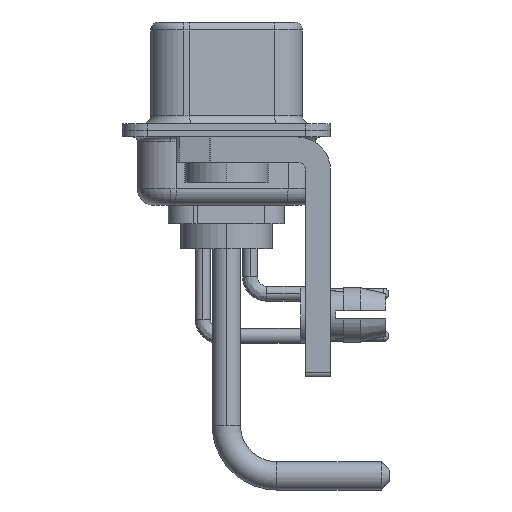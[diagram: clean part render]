
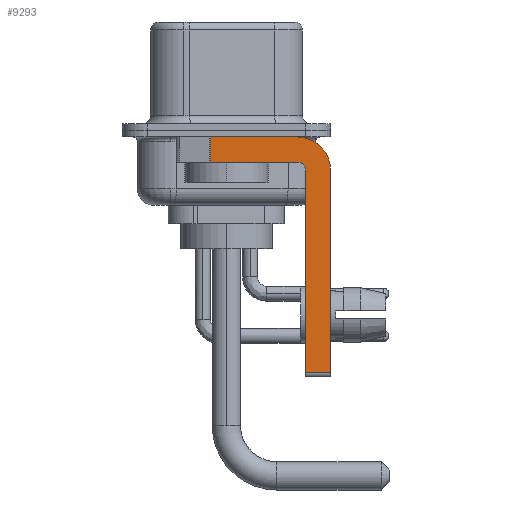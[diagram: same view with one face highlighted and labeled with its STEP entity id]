
A CAD part, left-side view. The second image highlights one B-rep face of the part: STEP entity #9293.
In plain terms, the highlighted planar face has unit normal (-1, 0, 0).
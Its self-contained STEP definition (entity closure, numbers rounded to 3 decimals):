
#61 = EDGE_CURVE ( 'NONE', #10969, #11477, #388, .T. ) ;
#388 = CIRCLE ( 'NONE', #13683, 2. ) ;
#877 = EDGE_CURVE ( 'NONE', #21684, #4207, #8972, .T. ) ;
#1241 = VERTEX_POINT ( 'NONE', #18661 ) ;
#1618 = CARTESIAN_POINT ( 'NONE',  ( -2.9, 0.978, -1.9 ) ) ;
#1762 = CARTESIAN_POINT ( 'NONE',  ( -2.9, -4.75, -14.8 ) ) ;
#1951 = DIRECTION ( 'NONE',  ( 1., 0., 0. ) ) ;
#2374 = VECTOR ( 'NONE', #17192, 1000. ) ;
#2614 = CIRCLE ( 'NONE', #9838, 0.5 ) ;
#2779 = DIRECTION ( 'NONE',  ( 1., 0., 0. ) ) ;
#2780 = DIRECTION ( 'NONE',  ( 0., 1., 0. ) ) ;
#2795 = EDGE_LOOP ( 'NONE', ( #20848, #18134, #19923, #14356, #10667, #23941, #11765, #3716 ) ) ;
#2895 = EDGE_CURVE ( 'NONE', #1241, #10969, #12571, .T. ) ;
#2924 = VERTEX_POINT ( 'NONE', #18760 ) ;
#3509 = LINE ( 'NONE', #1618, #22342 ) ;
#3649 = VECTOR ( 'NONE', #8600, 1000. ) ;
#3716 = ORIENTED_EDGE ( 'NONE', *, *, #61, .F. ) ;
#4207 = VERTEX_POINT ( 'NONE', #20794 ) ;
#4671 = PLANE ( 'NONE',  #16330 ) ;
#5119 = DIRECTION ( 'NONE',  ( 0., 0., -1. ) ) ;
#5318 = CARTESIAN_POINT ( 'NONE',  ( -2.9, -4.25, -2.4 ) ) ;
#5520 = DIRECTION ( 'NONE',  ( 0., 0., -1. ) ) ;
#6160 = LINE ( 'NONE', #17691, #10053 ) ;
#6886 = CARTESIAN_POINT ( 'NONE',  ( -2.9, -4.25, -0.4 ) ) ;
#7486 = CARTESIAN_POINT ( 'NONE',  ( -2.9, -4.25, -2.4 ) ) ;
#7518 = CARTESIAN_POINT ( 'NONE',  ( -2.9, -4.75, -2.4 ) ) ;
#8600 = DIRECTION ( 'NONE',  ( 0., -1., 0. ) ) ;
#8929 = EDGE_CURVE ( 'NONE', #21684, #9445, #22642, .T. ) ;
#8972 = LINE ( 'NONE', #18475, #3649 ) ;
#8979 = CARTESIAN_POINT ( 'NONE',  ( -2.9, 0.978, -1.9 ) ) ;
#9293 = ADVANCED_FACE ( 'NONE', ( #19837 ), #4671, .F. ) ;
#9445 = VERTEX_POINT ( 'NONE', #7518 ) ;
#9492 = CARTESIAN_POINT ( 'NONE',  ( -2.9, -6.25, -2.4 ) ) ;
#9838 = AXIS2_PLACEMENT_3D ( 'NONE', #5318, #22523, #13264 ) ;
#10053 = VECTOR ( 'NONE', #2780, 1000. ) ;
#10667 = ORIENTED_EDGE ( 'NONE', *, *, #8929, .F. ) ;
#10969 = VERTEX_POINT ( 'NONE', #6886 ) ;
#11477 = VERTEX_POINT ( 'NONE', #13812 ) ;
#11765 = ORIENTED_EDGE ( 'NONE', *, *, #19631, .F. ) ;
#12335 = EDGE_CURVE ( 'NONE', #1241, #24235, #3509, .T. ) ;
#12571 = LINE ( 'NONE', #20292, #13807 ) ;
#13264 = DIRECTION ( 'NONE',  ( 0., 0., 1. ) ) ;
#13683 = AXIS2_PLACEMENT_3D ( 'NONE', #7486, #1951, #24623 ) ;
#13807 = VECTOR ( 'NONE', #18024, 1000. ) ;
#13812 = CARTESIAN_POINT ( 'NONE',  ( -2.9, -6.25, -2.4 ) ) ;
#14356 = ORIENTED_EDGE ( 'NONE', *, *, #15057, .F. ) ;
#14475 = VECTOR ( 'NONE', #5119, 1000. ) ;
#14623 = CARTESIAN_POINT ( 'NONE',  ( -2.9, -4.75, -14.55 ) ) ;
#15057 = EDGE_CURVE ( 'NONE', #9445, #2924, #2614, .T. ) ;
#16330 = AXIS2_PLACEMENT_3D ( 'NONE', #20088, #2779, #18209 ) ;
#17192 = DIRECTION ( 'NONE',  ( 0., 0., 1. ) ) ;
#17691 = CARTESIAN_POINT ( 'NONE',  ( -2.9, -4.25, -1.9 ) ) ;
#18024 = DIRECTION ( 'NONE',  ( 0., -1., 0. ) ) ;
#18134 = ORIENTED_EDGE ( 'NONE', *, *, #12335, .T. ) ;
#18209 = DIRECTION ( 'NONE',  ( 0., 0., -1. ) ) ;
#18475 = CARTESIAN_POINT ( 'NONE',  ( -2.9, -4.25, -14.55 ) ) ;
#18661 = CARTESIAN_POINT ( 'NONE',  ( -2.9, 0.978, -0.4 ) ) ;
#18760 = CARTESIAN_POINT ( 'NONE',  ( -2.9, -4.25, -1.9 ) ) ;
#19631 = EDGE_CURVE ( 'NONE', #11477, #4207, #22453, .T. ) ;
#19837 = FACE_OUTER_BOUND ( 'NONE', #2795, .T. ) ;
#19923 = ORIENTED_EDGE ( 'NONE', *, *, #21555, .F. ) ;
#20088 = CARTESIAN_POINT ( 'NONE',  ( -2.9, -4.25, -2.4 ) ) ;
#20292 = CARTESIAN_POINT ( 'NONE',  ( -2.9, 3., -0.4 ) ) ;
#20794 = CARTESIAN_POINT ( 'NONE',  ( -2.9, -6.25, -14.55 ) ) ;
#20848 = ORIENTED_EDGE ( 'NONE', *, *, #2895, .F. ) ;
#21555 = EDGE_CURVE ( 'NONE', #2924, #24235, #6160, .T. ) ;
#21684 = VERTEX_POINT ( 'NONE', #14623 ) ;
#22342 = VECTOR ( 'NONE', #5520, 1000. ) ;
#22453 = LINE ( 'NONE', #9492, #14475 ) ;
#22523 = DIRECTION ( 'NONE',  ( -1., 0., 0. ) ) ;
#22642 = LINE ( 'NONE', #1762, #2374 ) ;
#23941 = ORIENTED_EDGE ( 'NONE', *, *, #877, .T. ) ;
#24235 = VERTEX_POINT ( 'NONE', #8979 ) ;
#24623 = DIRECTION ( 'NONE',  ( 0., 0., -1. ) ) ;
